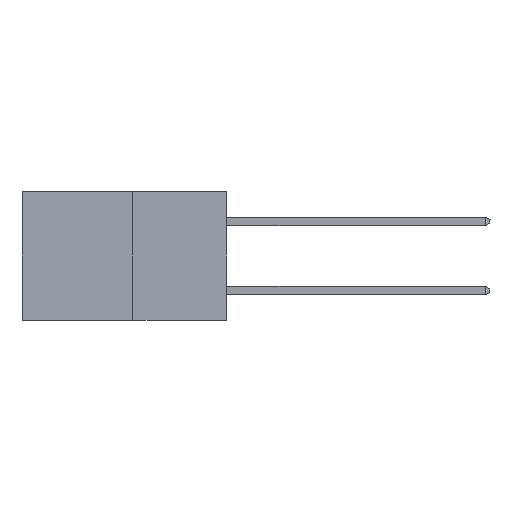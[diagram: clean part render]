
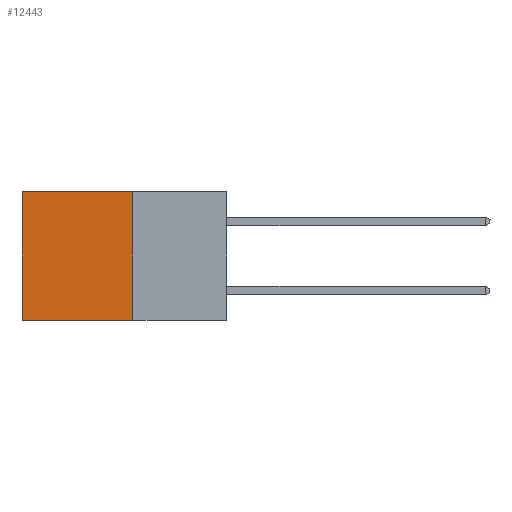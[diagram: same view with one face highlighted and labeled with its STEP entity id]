
A CAD part, left-side view. The second image highlights one B-rep face of the part: STEP entity #12443.
In plain terms, the highlighted planar face has unit normal (-1, 0, 0).
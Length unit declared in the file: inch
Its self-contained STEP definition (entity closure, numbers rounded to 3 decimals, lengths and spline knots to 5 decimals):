
#95 = LINE ( 'NONE', #1310, #13378 ) ;
#169 = DIRECTION ( 'NONE',  ( 0., 0., -1. ) ) ;
#456 = LINE ( 'NONE', #15499, #6863 ) ;
#525 = DIRECTION ( 'NONE',  ( 0., 0., -1. ) ) ;
#682 = VECTOR ( 'NONE', #169, 39.37008 ) ;
#1106 = VERTEX_POINT ( 'NONE', #8941 ) ;
#1310 = CARTESIAN_POINT ( 'NONE',  ( 0.277, 0.27, -0.37 ) ) ;
#1941 = VERTEX_POINT ( 'NONE', #8918 ) ;
#1942 = FACE_OUTER_BOUND ( 'NONE', #15115, .T. ) ;
#2146 = EDGE_CURVE ( 'NONE', #1106, #5764, #456, .T. ) ;
#3277 = EDGE_CURVE ( 'NONE', #1941, #5764, #4024, .T. ) ;
#4024 = LINE ( 'NONE', #6515, #682 ) ;
#4119 = VECTOR ( 'NONE', #11075, 39.37008 ) ;
#4156 = DIRECTION ( 'NONE',  ( 1., 0., 0. ) ) ;
#4276 = VERTEX_POINT ( 'NONE', #6879 ) ;
#4509 = CARTESIAN_POINT ( 'NONE',  ( 0.277, 0.27, 0. ) ) ;
#5764 = VERTEX_POINT ( 'NONE', #12270 ) ;
#6515 = CARTESIAN_POINT ( 'NONE',  ( 0.277, 0.59, -0.37 ) ) ;
#6740 = CARTESIAN_POINT ( 'NONE',  ( 0.277, 0.27, -0.37 ) ) ;
#6863 = VECTOR ( 'NONE', #15449, 39.37008 ) ;
#6879 = CARTESIAN_POINT ( 'NONE',  ( 0.277, 0.27, 0. ) ) ;
#7314 = ORIENTED_EDGE ( 'NONE', *, *, #3277, .T. ) ;
#7592 = AXIS2_PLACEMENT_3D ( 'NONE', #6740, #4156, #13294 ) ;
#8918 = CARTESIAN_POINT ( 'NONE',  ( 0.277, 0.59, 0. ) ) ;
#8941 = CARTESIAN_POINT ( 'NONE',  ( 0.277, 0.27, -0.37 ) ) ;
#9108 = ORIENTED_EDGE ( 'NONE', *, *, #2146, .F. ) ;
#9156 = ORIENTED_EDGE ( 'NONE', *, *, #10348, .F. ) ;
#9512 = ORIENTED_EDGE ( 'NONE', *, *, #12515, .T. ) ;
#10348 = EDGE_CURVE ( 'NONE', #4276, #1106, #95, .T. ) ;
#11075 = DIRECTION ( 'NONE',  ( 0., 1., 0. ) ) ;
#12028 = PLANE ( 'NONE',  #7592 ) ;
#12270 = CARTESIAN_POINT ( 'NONE',  ( 0.277, 0.59, -0.37 ) ) ;
#12443 = ADVANCED_FACE ( 'NONE', ( #1942 ), #12028, .F. ) ;
#12515 = EDGE_CURVE ( 'NONE', #4276, #1941, #14443, .T. ) ;
#13294 = DIRECTION ( 'NONE',  ( 0., 0., -1. ) ) ;
#13378 = VECTOR ( 'NONE', #525, 39.37008 ) ;
#14443 = LINE ( 'NONE', #4509, #4119 ) ;
#15115 = EDGE_LOOP ( 'NONE', ( #7314, #9108, #9156, #9512 ) ) ;
#15449 = DIRECTION ( 'NONE',  ( 0., 1., 0. ) ) ;
#15499 = CARTESIAN_POINT ( 'NONE',  ( 0.277, 0.27, -0.37 ) ) ;
